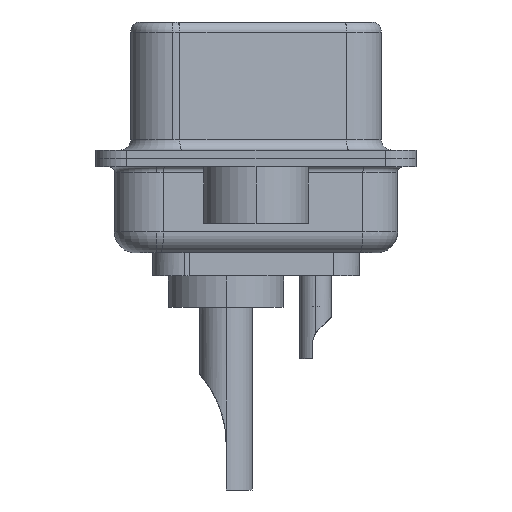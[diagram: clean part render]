
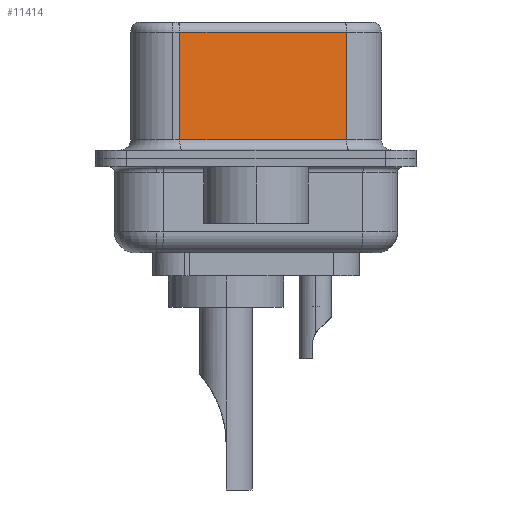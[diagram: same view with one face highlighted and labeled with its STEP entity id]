
A CAD part, left-side view. The second image highlights one B-rep face of the part: STEP entity #11414.
In plain terms, the highlighted planar face has unit normal (-0.985, -0.174, 0).
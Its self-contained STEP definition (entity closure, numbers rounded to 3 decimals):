
#287 = VERTEX_POINT ( 'NONE', #6266 ) ;
#444 = DIRECTION ( 'NONE',  ( -0.174, 0.985, 0. ) ) ;
#1080 = VERTEX_POINT ( 'NONE', #20051 ) ;
#1717 = VECTOR ( 'NONE', #444, 1000. ) ;
#2714 = LINE ( 'NONE', #4299, #10909 ) ;
#2977 = EDGE_CURVE ( 'NONE', #10490, #8423, #6233, .T. ) ;
#4299 = CARTESIAN_POINT ( 'NONE',  ( 5.132, -4.322, 0.9 ) ) ;
#5972 = DIRECTION ( 'NONE',  ( 0.174, -0.985, 0. ) ) ;
#6233 = LINE ( 'NONE', #21105, #13778 ) ;
#6241 = LINE ( 'NONE', #15244, #1717 ) ;
#6266 = CARTESIAN_POINT ( 'NONE',  ( 3.73, 3.628, 6.02 ) ) ;
#7012 = CARTESIAN_POINT ( 'NONE',  ( 5.132, -4.322, 6.52 ) ) ;
#7080 = PLANE ( 'NONE',  #11344 ) ;
#7994 = FACE_OUTER_BOUND ( 'NONE', #16272, .T. ) ;
#8116 = DIRECTION ( 'NONE',  ( 0., 0., -1. ) ) ;
#8423 = VERTEX_POINT ( 'NONE', #20253 ) ;
#8650 = DIRECTION ( 'NONE',  ( 0.985, 0.174, 0. ) ) ;
#8825 = CARTESIAN_POINT ( 'NONE',  ( 5.132, -4.322, 6.02 ) ) ;
#10297 = ORIENTED_EDGE ( 'NONE', *, *, #2977, .F. ) ;
#10490 = VERTEX_POINT ( 'NONE', #8825 ) ;
#10909 = VECTOR ( 'NONE', #5972, 1000. ) ;
#11293 = LINE ( 'NONE', #14754, #20066 ) ;
#11344 = AXIS2_PLACEMENT_3D ( 'NONE', #7012, #8650, #20105 ) ;
#11414 = ADVANCED_FACE ( 'NONE', ( #7994 ), #7080, .F. ) ;
#13778 = VECTOR ( 'NONE', #8116, 1000. ) ;
#14754 = CARTESIAN_POINT ( 'NONE',  ( 3.73, 3.628, 6.52 ) ) ;
#14909 = ORIENTED_EDGE ( 'NONE', *, *, #20364, .T. ) ;
#15244 = CARTESIAN_POINT ( 'NONE',  ( 5.132, -4.322, 6.02 ) ) ;
#15334 = ORIENTED_EDGE ( 'NONE', *, *, #21044, .T. ) ;
#16272 = EDGE_LOOP ( 'NONE', ( #10297, #15334, #14909, #21101 ) ) ;
#16586 = EDGE_CURVE ( 'NONE', #1080, #8423, #2714, .T. ) ;
#18018 = DIRECTION ( 'NONE',  ( 0., 0., -1. ) ) ;
#20051 = CARTESIAN_POINT ( 'NONE',  ( 3.73, 3.628, 0.9 ) ) ;
#20066 = VECTOR ( 'NONE', #18018, 1000. ) ;
#20105 = DIRECTION ( 'NONE',  ( -0.174, 0.985, 0. ) ) ;
#20253 = CARTESIAN_POINT ( 'NONE',  ( 5.132, -4.322, 0.9 ) ) ;
#20364 = EDGE_CURVE ( 'NONE', #287, #1080, #11293, .T. ) ;
#21044 = EDGE_CURVE ( 'NONE', #10490, #287, #6241, .T. ) ;
#21101 = ORIENTED_EDGE ( 'NONE', *, *, #16586, .T. ) ;
#21105 = CARTESIAN_POINT ( 'NONE',  ( 5.132, -4.322, 6.52 ) ) ;
